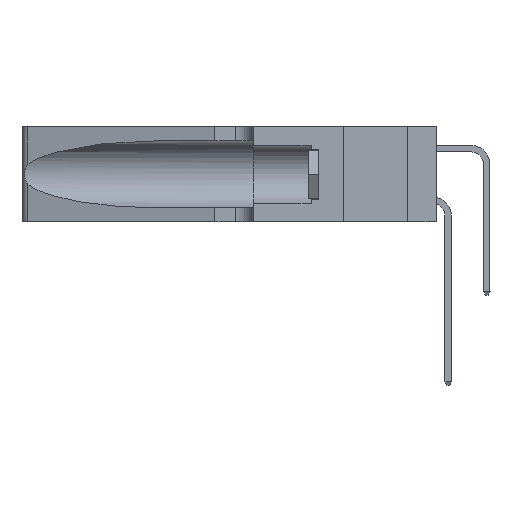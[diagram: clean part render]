
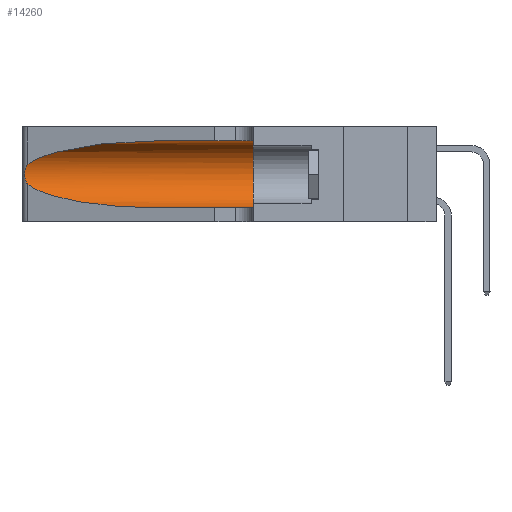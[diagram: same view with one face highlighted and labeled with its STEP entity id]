
A CAD part, left-side view. The second image highlights one B-rep face of the part: STEP entity #14260.
In plain terms, the highlighted cylindrical face has radius 3.308 mm (diameter 6.617 mm), a partial arc.
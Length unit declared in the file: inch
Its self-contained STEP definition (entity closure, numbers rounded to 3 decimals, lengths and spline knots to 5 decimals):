
#3 = ORIENTED_EDGE ( 'NONE', *, *, #12048, .F. ) ;
#53 = CARTESIAN_POINT ( 'NONE',  ( 0.18966, 0.96281, 0.31525 ) ) ;
#771 = ORIENTED_EDGE ( 'NONE', *, *, #30112, .T. ) ;
#1309 = CARTESIAN_POINT ( 'NONE',  ( 0.25487, 1.22718, 0.22369 ) ) ;
#1323 = VERTEX_POINT ( 'NONE', #14044 ) ;
#2108 = VERTEX_POINT ( 'NONE', #5845 ) ;
#2301 = EDGE_CURVE ( 'NONE', #27662, #11057, #5203, .T. ) ;
#3332 = DIRECTION ( 'NONE',  ( 0., 0., 1. ) ) ;
#3830 = CARTESIAN_POINT ( 'NONE',  ( 0.1305, 0.35, 0.31525 ) ) ;
#4765 = CARTESIAN_POINT ( 'NONE',  ( 0.1305, 0.35, 0.05475 ) ) ;
#4991 = EDGE_CURVE ( 'NONE', #26977, #11057, #10452, .T. ) ;
#5203 = LINE ( 'NONE', #9107, #9433 ) ;
#5845 = CARTESIAN_POINT ( 'NONE',  ( 0.1305, 0.72297, 0.31525 ) ) ;
#5952 = CARTESIAN_POINT ( 'NONE',  ( 0.26075, 1.23896, 0.19203 ) ) ;
#6059 = CARTESIAN_POINT ( 'NONE',  ( 0.25487, 1.22718, 0.14631 ) ) ;
#7075 = AXIS2_PLACEMENT_3D ( 'NONE', #28800, #9079, #26444 ) ;
#7943 = CYLINDRICAL_SURFACE ( 'NONE', #7075, 0.13025 ) ;
#8552 = CARTESIAN_POINT ( 'NONE',  ( 0.1305, 1.61858, 0.31525 ) ) ;
#8611 = CARTESIAN_POINT ( 'NONE',  ( 0.25639, 1.23186, 0.15144 ) ) ;
#9079 = DIRECTION ( 'NONE',  ( 0., -1., 0. ) ) ;
#9107 = CARTESIAN_POINT ( 'NONE',  ( 0.1305, 1.61858, 0.05475 ) ) ;
#9433 = VECTOR ( 'NONE', #21008, 39.37008 ) ;
#9724 = CARTESIAN_POINT ( 'NONE',  ( 0.25487, 1.22718, 0.14631 ) ) ;
#10452 = CIRCLE ( 'NONE', #11602, 0.13025 ) ;
#10870 = CARTESIAN_POINT ( 'NONE',  ( 0.25555, 1.22993, 0.14849 ) ) ;
#11057 = VERTEX_POINT ( 'NONE', #4765 ) ;
#11181 = CARTESIAN_POINT ( 'NONE',  ( 0.26075, 1.23896, 0.178 ) ) ;
#11602 = AXIS2_PLACEMENT_3D ( 'NONE', #15455, #15565, #3332 ) ;
#12048 = EDGE_CURVE ( 'NONE', #2108, #26977, #14594, .T. ) ;
#13247 = CARTESIAN_POINT ( 'NONE',  ( 0.26017, 1.23833, 0.17102 ) ) ;
#13805 = ORIENTED_EDGE ( 'NONE', *, *, #2301, .T. ) ;
#14044 = CARTESIAN_POINT ( 'NONE',  ( 0.25487, 1.22718, 0.14631 ) ) ;
#14205 = VECTOR ( 'NONE', #20762, 39.37008 ) ;
#14243 = EDGE_LOOP ( 'NONE', ( #19787, #771, #27138, #13805, #26640, #3 ) ) ;
#14260 = ADVANCED_FACE ( 'NONE', ( #16777 ), #7943, .F. ) ;
#14403 = EDGE_CURVE ( 'NONE', #2108, #23486, #25142, .T. ) ;
#14594 = LINE ( 'NONE', #8552, #14205 ) ;
#14755 = CARTESIAN_POINT ( 'NONE',  ( 0.1305, 0.72297, 0.31525 ) ) ;
#14972 = CARTESIAN_POINT ( 'NONE',  ( 0.1305, 0.72297, 0.05475 ) ) ;
#15455 = CARTESIAN_POINT ( 'NONE',  ( 0.1305, 0.35, 0.185 ) ) ;
#15565 = DIRECTION ( 'NONE',  ( 0., 1., 0. ) ) ;
#15783 = CARTESIAN_POINT ( 'NONE',  ( 0.25789, 1.23486, 0.15765 ) ) ;
#16777 = FACE_OUTER_BOUND ( 'NONE', #14243, .T. ) ;
#17194 = CARTESIAN_POINT ( 'NONE',  ( 0.25487, 1.22718, 0.22369 ) ) ;
#17526 = CARTESIAN_POINT ( 'NONE',  ( 0.18966, 0.96281, 0.05475 ) ) ;
#18038 = B_SPLINE_CURVE_WITH_KNOTS ( 'NONE', 3,
 ( #1309, #25980, #27912, #20716, #25879, #30765, #5952, #11181, #13247, #30337, #15783, #8611, #10870, #6059 ),
 .UNSPECIFIED., .F., .F.,
 ( 4, 2, 2, 2, 2, 2, 4 ),
 ( 0., 0.00027, 0.00053, 0.00107, 0.0016, 0.00187, 0.00214 ),
 .UNSPECIFIED. ) ;
#19355 = CARTESIAN_POINT ( 'NONE',  ( 0.2373, 1.15595, 0.28018 ) ) ;
#19786 = CARTESIAN_POINT ( 'NONE',  ( 0.2373, 1.15595, 0.08982 ) ) ;
#19787 = ORIENTED_EDGE ( 'NONE', *, *, #14403, .T. ) ;
#20716 = CARTESIAN_POINT ( 'NONE',  ( 0.25787, 1.23484, 0.2124 ) ) ;
#20762 = DIRECTION ( 'NONE',  ( 0., -1., 0. ) ) ;
#20960 = CARTESIAN_POINT ( 'NONE',  ( 0.1305, 0.72297, 0.05475 ) ) ;
#21008 = DIRECTION ( 'NONE',  ( 0., -1., 0. ) ) ;
#22026 = CARTESIAN_POINT ( 'NONE',  ( 0.25487, 1.22718, 0.22369 ) ) ;
#23486 = VERTEX_POINT ( 'NONE', #22026 ) ;
#25142 =( BOUNDED_CURVE ( )  B_SPLINE_CURVE ( 3, ( #14755, #53, #19355, #17194 ),
 .UNSPECIFIED., .F., .T. ) 
 B_SPLINE_CURVE_WITH_KNOTS ( ( 4, 4 ),
 ( 1.5708, 2.84003 ),
 .UNSPECIFIED. ) 
 CURVE ( )  GEOMETRIC_REPRESENTATION_ITEM ( )  RATIONAL_B_SPLINE_CURVE ( ( 1., 0.87, 0.87, 1. ) ) 
 REPRESENTATION_ITEM ( '' )  );
#25279 = EDGE_CURVE ( 'NONE', #1323, #27662, #29438, .T. ) ;
#25879 = CARTESIAN_POINT ( 'NONE',  ( 0.25854, 1.2359, 0.20912 ) ) ;
#25980 = CARTESIAN_POINT ( 'NONE',  ( 0.25555, 1.22994, 0.2215 ) ) ;
#26444 = DIRECTION ( 'NONE',  ( 0., 0., -1. ) ) ;
#26640 = ORIENTED_EDGE ( 'NONE', *, *, #4991, .F. ) ;
#26977 = VERTEX_POINT ( 'NONE', #3830 ) ;
#27138 = ORIENTED_EDGE ( 'NONE', *, *, #25279, .T. ) ;
#27662 = VERTEX_POINT ( 'NONE', #20960 ) ;
#27912 = CARTESIAN_POINT ( 'NONE',  ( 0.25639, 1.23184, 0.21858 ) ) ;
#28800 = CARTESIAN_POINT ( 'NONE',  ( 0.1305, 1.61858, 0.185 ) ) ;
#29438 =( BOUNDED_CURVE ( )  B_SPLINE_CURVE ( 3, ( #9724, #19786, #17526, #14972 ),
 .UNSPECIFIED., .F., .T. ) 
 B_SPLINE_CURVE_WITH_KNOTS ( ( 4, 4 ),
 ( 3.44316, 4.71239 ),
 .UNSPECIFIED. ) 
 CURVE ( )  GEOMETRIC_REPRESENTATION_ITEM ( )  RATIONAL_B_SPLINE_CURVE ( ( 1., 0.87, 0.87, 1. ) ) 
 REPRESENTATION_ITEM ( '' )  );
#30112 = EDGE_CURVE ( 'NONE', #23486, #1323, #18038, .T. ) ;
#30337 = CARTESIAN_POINT ( 'NONE',  ( 0.25856, 1.23593, 0.16098 ) ) ;
#30765 = CARTESIAN_POINT ( 'NONE',  ( 0.26018, 1.23835, 0.19895 ) ) ;
